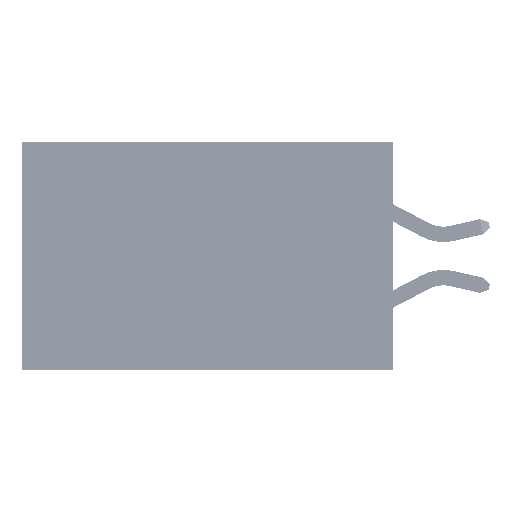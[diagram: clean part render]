
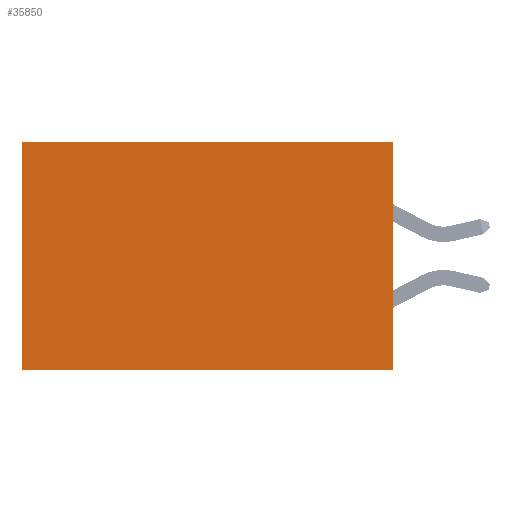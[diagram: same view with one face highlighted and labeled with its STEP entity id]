
A CAD part, left-side view. The second image highlights one B-rep face of the part: STEP entity #35850.
In plain terms, the highlighted planar face has unit normal (-1, 0, 0).
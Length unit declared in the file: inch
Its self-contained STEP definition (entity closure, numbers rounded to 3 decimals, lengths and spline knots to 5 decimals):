
#242 = VECTOR ( 'NONE', #18715, 39.37008 ) ;
#447 = EDGE_CURVE ( 'NONE', #29759, #37888, #16006, .T. ) ;
#1365 = LINE ( 'NONE', #11671, #242 ) ;
#2257 = VERTEX_POINT ( 'NONE', #14053 ) ;
#3417 = EDGE_LOOP ( 'NONE', ( #12844, #10669, #15772, #28005 ) ) ;
#5764 = EDGE_CURVE ( 'NONE', #2257, #37888, #11113, .T. ) ;
#6658 = VECTOR ( 'NONE', #39845, 39.37008 ) ;
#10669 = ORIENTED_EDGE ( 'NONE', *, *, #5764, .F. ) ;
#11113 = LINE ( 'NONE', #34316, #37855 ) ;
#11671 = CARTESIAN_POINT ( 'NONE',  ( 0.2875, 0., 0. ) ) ;
#12786 = EDGE_CURVE ( 'NONE', #44774, #29759, #29732, .T. ) ;
#12844 = ORIENTED_EDGE ( 'NONE', *, *, #447, .T. ) ;
#13326 = DIRECTION ( 'NONE',  ( 0., 0., -1. ) ) ;
#14053 = CARTESIAN_POINT ( 'NONE',  ( 0.2875, 0., -0.37 ) ) ;
#15772 = ORIENTED_EDGE ( 'NONE', *, *, #24762, .F. ) ;
#15910 = CARTESIAN_POINT ( 'NONE',  ( 0.2875, 0., 0. ) ) ;
#16006 = LINE ( 'NONE', #22788, #6658 ) ;
#18715 = DIRECTION ( 'NONE',  ( 0., 0., -1. ) ) ;
#20455 = DIRECTION ( 'NONE',  ( 0., 1., 0. ) ) ;
#21770 = CARTESIAN_POINT ( 'NONE',  ( 0.2875, 0., 0. ) ) ;
#22788 = CARTESIAN_POINT ( 'NONE',  ( 0.2875, 0.6, 0. ) ) ;
#24762 = EDGE_CURVE ( 'NONE', #44774, #2257, #1365, .T. ) ;
#28005 = ORIENTED_EDGE ( 'NONE', *, *, #12786, .T. ) ;
#28633 = VECTOR ( 'NONE', #36933, 39.37008 ) ;
#29732 = LINE ( 'NONE', #15910, #28633 ) ;
#29759 = VERTEX_POINT ( 'NONE', #32884 ) ;
#30769 = PLANE ( 'NONE',  #31728 ) ;
#31703 = FACE_OUTER_BOUND ( 'NONE', #3417, .T. ) ;
#31728 = AXIS2_PLACEMENT_3D ( 'NONE', #37412, #34231, #13326 ) ;
#32113 = CARTESIAN_POINT ( 'NONE',  ( 0.2875, 0.6, -0.37 ) ) ;
#32884 = CARTESIAN_POINT ( 'NONE',  ( 0.2875, 0.6, 0. ) ) ;
#34231 = DIRECTION ( 'NONE',  ( 1., 0., 0. ) ) ;
#34316 = CARTESIAN_POINT ( 'NONE',  ( 0.2875, 0., -0.37 ) ) ;
#35850 = ADVANCED_FACE ( 'NONE', ( #31703 ), #30769, .F. ) ;
#36933 = DIRECTION ( 'NONE',  ( 0., 1., 0. ) ) ;
#37412 = CARTESIAN_POINT ( 'NONE',  ( 0.2875, 0., 0. ) ) ;
#37855 = VECTOR ( 'NONE', #20455, 39.37008 ) ;
#37888 = VERTEX_POINT ( 'NONE', #32113 ) ;
#39845 = DIRECTION ( 'NONE',  ( 0., 0., -1. ) ) ;
#44774 = VERTEX_POINT ( 'NONE', #21770 ) ;
